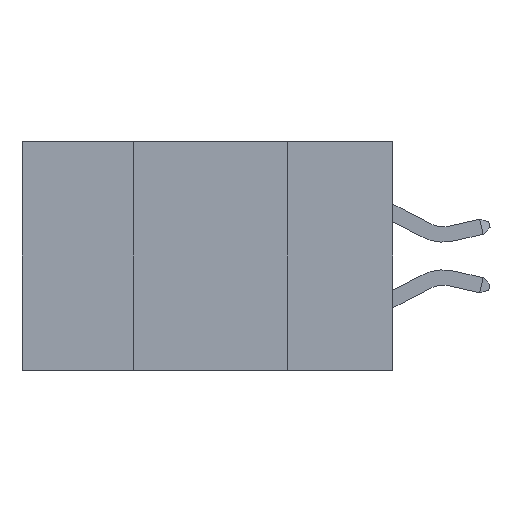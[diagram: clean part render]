
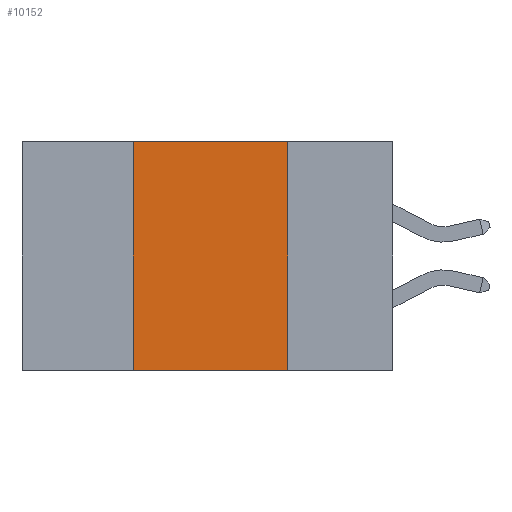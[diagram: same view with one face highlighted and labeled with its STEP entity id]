
A CAD part, left-side view. The second image highlights one B-rep face of the part: STEP entity #10152.
In plain terms, the highlighted planar face has unit normal (-1, 0, 0).
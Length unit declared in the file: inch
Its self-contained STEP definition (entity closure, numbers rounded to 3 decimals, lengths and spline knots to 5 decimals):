
#496 = CARTESIAN_POINT ( 'NONE',  ( 0., 0.17, 0. ) ) ;
#1632 = CARTESIAN_POINT ( 'NONE',  ( 0., 0.17, -0.37 ) ) ;
#1691 = PLANE ( 'NONE',  #19268 ) ;
#2578 = EDGE_LOOP ( 'NONE', ( #15582, #12162, #4301, #18901 ) ) ;
#3739 = DIRECTION ( 'NONE',  ( 0., -1., 0. ) ) ;
#4301 = ORIENTED_EDGE ( 'NONE', *, *, #18039, .F. ) ;
#4326 = VERTEX_POINT ( 'NONE', #5683 ) ;
#4961 = DIRECTION ( 'NONE',  ( 0., -1., 0. ) ) ;
#5287 = DIRECTION ( 'NONE',  ( 0., 0., -1. ) ) ;
#5683 = CARTESIAN_POINT ( 'NONE',  ( 0., 0.42, -0.37 ) ) ;
#5929 = DIRECTION ( 'NONE',  ( 0., 0., 1. ) ) ;
#5937 = EDGE_CURVE ( 'NONE', #7267, #15937, #20599, .T. ) ;
#6001 = CARTESIAN_POINT ( 'NONE',  ( 0., 0.42, 0. ) ) ;
#6571 = CARTESIAN_POINT ( 'NONE',  ( 0., 0.42, 0. ) ) ;
#7267 = VERTEX_POINT ( 'NONE', #10976 ) ;
#8413 = EDGE_CURVE ( 'NONE', #10002, #7267, #16238, .T. ) ;
#8838 = CARTESIAN_POINT ( 'NONE',  ( 0., 0.6, 0. ) ) ;
#9590 = FACE_OUTER_BOUND ( 'NONE', #2578, .T. ) ;
#10002 = VERTEX_POINT ( 'NONE', #6571 ) ;
#10152 = ADVANCED_FACE ( 'NONE', ( #9590 ), #1691, .F. ) ;
#10976 = CARTESIAN_POINT ( 'NONE',  ( 0., 0.17, 0. ) ) ;
#11153 = VECTOR ( 'NONE', #4961, 39.37008 ) ;
#12162 = ORIENTED_EDGE ( 'NONE', *, *, #8413, .F. ) ;
#12726 = LINE ( 'NONE', #6001, #17570 ) ;
#13253 = CARTESIAN_POINT ( 'NONE',  ( 0., 0.6, -0.37 ) ) ;
#15205 = EDGE_CURVE ( 'NONE', #4326, #15937, #20300, .T. ) ;
#15221 = DIRECTION ( 'NONE',  ( 1., 0., 0. ) ) ;
#15582 = ORIENTED_EDGE ( 'NONE', *, *, #5937, .F. ) ;
#15937 = VERTEX_POINT ( 'NONE', #1632 ) ;
#16238 = LINE ( 'NONE', #8838, #20012 ) ;
#16697 = CARTESIAN_POINT ( 'NONE',  ( 0., 0.6, 0. ) ) ;
#16850 = DIRECTION ( 'NONE',  ( 0., 0., -1. ) ) ;
#17570 = VECTOR ( 'NONE', #5929, 39.37008 ) ;
#18039 = EDGE_CURVE ( 'NONE', #4326, #10002, #12726, .T. ) ;
#18901 = ORIENTED_EDGE ( 'NONE', *, *, #15205, .T. ) ;
#19268 = AXIS2_PLACEMENT_3D ( 'NONE', #16697, #15221, #5287 ) ;
#20012 = VECTOR ( 'NONE', #3739, 39.37008 ) ;
#20096 = VECTOR ( 'NONE', #16850, 39.37008 ) ;
#20300 = LINE ( 'NONE', #13253, #11153 ) ;
#20599 = LINE ( 'NONE', #496, #20096 ) ;
